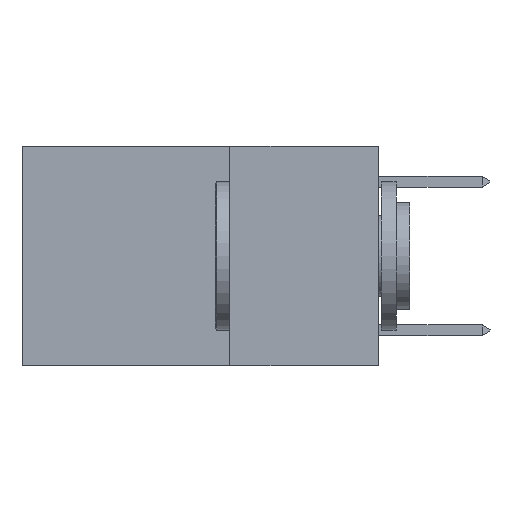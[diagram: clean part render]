
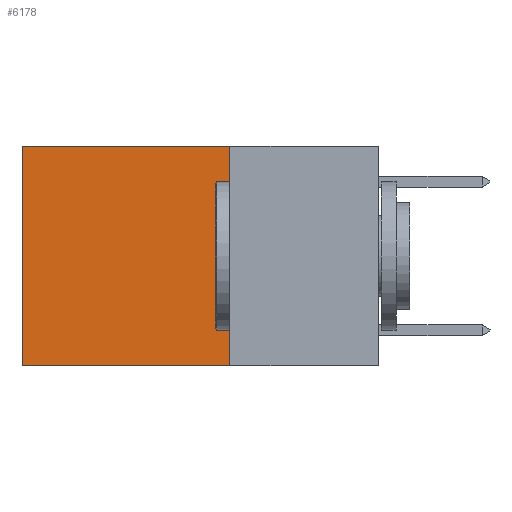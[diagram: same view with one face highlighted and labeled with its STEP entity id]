
A CAD part, left-side view. The second image highlights one B-rep face of the part: STEP entity #6178.
In plain terms, the highlighted planar face has unit normal (-1, 0, 0).
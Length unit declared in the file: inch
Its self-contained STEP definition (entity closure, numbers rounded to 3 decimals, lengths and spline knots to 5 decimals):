
#86 = LINE ( 'NONE', #10260, #321 ) ;
#321 = VECTOR ( 'NONE', #10708, 39.37008 ) ;
#434 = DIRECTION ( 'NONE',  ( 0., 0., -1. ) ) ;
#623 = CARTESIAN_POINT ( 'NONE',  ( 0.2625, 0.25, -0.37 ) ) ;
#660 = CARTESIAN_POINT ( 'NONE',  ( 0.2625, 0.6, 0. ) ) ;
#1467 = CARTESIAN_POINT ( 'NONE',  ( 0.2625, 0.6, 0. ) ) ;
#2858 = DIRECTION ( 'NONE',  ( 0., 1., 0. ) ) ;
#4459 = EDGE_CURVE ( 'NONE', #13785, #5068, #14438, .T. ) ;
#5008 = EDGE_CURVE ( 'NONE', #13785, #17588, #86, .T. ) ;
#5068 = VERTEX_POINT ( 'NONE', #8823 ) ;
#6017 = CARTESIAN_POINT ( 'NONE',  ( 0.2625, 0.25, 0. ) ) ;
#6042 = AXIS2_PLACEMENT_3D ( 'NONE', #28002, #27602, #27541 ) ;
#6178 = ADVANCED_FACE ( 'NONE', ( #11785 ), #27824, .F. ) ;
#6784 = CARTESIAN_POINT ( 'NONE',  ( 0.2625, 0.6, -0.37 ) ) ;
#8823 = CARTESIAN_POINT ( 'NONE',  ( 0.2625, 0.25, -0.37 ) ) ;
#9472 = VERTEX_POINT ( 'NONE', #6784 ) ;
#9717 = VECTOR ( 'NONE', #2858, 39.37008 ) ;
#9846 = LINE ( 'NONE', #623, #9717 ) ;
#10164 = ORIENTED_EDGE ( 'NONE', *, *, #20279, .T. ) ;
#10260 = CARTESIAN_POINT ( 'NONE',  ( 0.2625, 0.25, 0. ) ) ;
#10708 = DIRECTION ( 'NONE',  ( 0., 1., 0. ) ) ;
#11785 = FACE_OUTER_BOUND ( 'NONE', #19935, .T. ) ;
#12179 = VECTOR ( 'NONE', #434, 39.37008 ) ;
#12311 = LINE ( 'NONE', #660, #12179 ) ;
#13785 = VERTEX_POINT ( 'NONE', #6017 ) ;
#14011 = ORIENTED_EDGE ( 'NONE', *, *, #28134, .F. ) ;
#14438 = LINE ( 'NONE', #19597, #15021 ) ;
#15021 = VECTOR ( 'NONE', #20399, 39.37008 ) ;
#17588 = VERTEX_POINT ( 'NONE', #1467 ) ;
#18597 = ORIENTED_EDGE ( 'NONE', *, *, #5008, .T. ) ;
#19399 = ORIENTED_EDGE ( 'NONE', *, *, #4459, .F. ) ;
#19597 = CARTESIAN_POINT ( 'NONE',  ( 0.2625, 0.25, 0. ) ) ;
#19935 = EDGE_LOOP ( 'NONE', ( #10164, #14011, #19399, #18597 ) ) ;
#20279 = EDGE_CURVE ( 'NONE', #17588, #9472, #12311, .T. ) ;
#20399 = DIRECTION ( 'NONE',  ( 0., 0., -1. ) ) ;
#27541 = DIRECTION ( 'NONE',  ( 0., 0., -1. ) ) ;
#27602 = DIRECTION ( 'NONE',  ( 1., 0., 0. ) ) ;
#27824 = PLANE ( 'NONE',  #6042 ) ;
#28002 = CARTESIAN_POINT ( 'NONE',  ( 0.2625, 0.25, 0. ) ) ;
#28134 = EDGE_CURVE ( 'NONE', #5068, #9472, #9846, .T. ) ;
